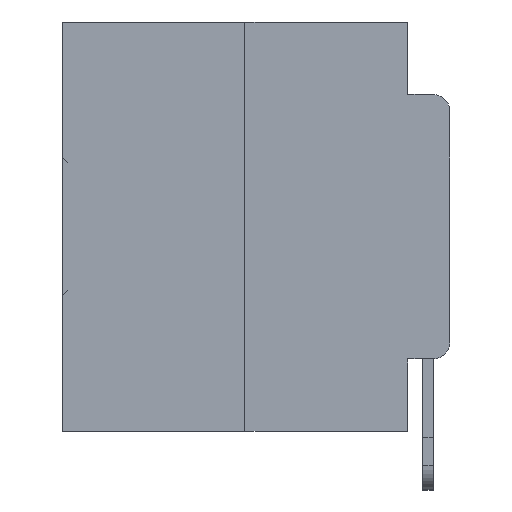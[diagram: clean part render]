
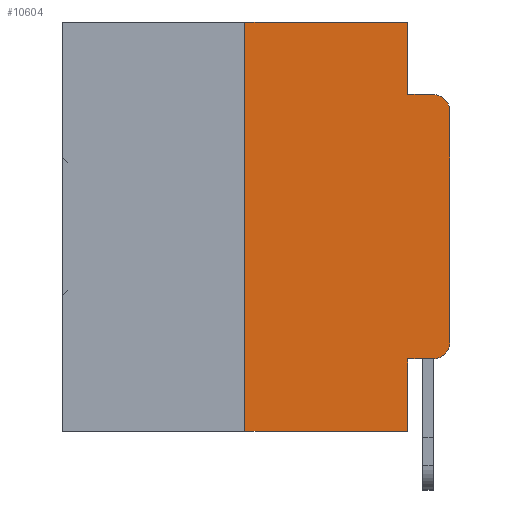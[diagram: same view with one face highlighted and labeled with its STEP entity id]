
A CAD part, left-side view. The second image highlights one B-rep face of the part: STEP entity #10604.
In plain terms, the highlighted planar face has unit normal (-1, 0, 0).
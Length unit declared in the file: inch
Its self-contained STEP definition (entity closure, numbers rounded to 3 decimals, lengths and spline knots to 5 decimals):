
#63 = LINE ( 'NONE', #8685, #33603 ) ;
#419 = DIRECTION ( 'NONE',  ( 0., -1., 0. ) ) ;
#886 = DIRECTION ( 'NONE',  ( 0., 0., -1. ) ) ;
#1869 = LINE ( 'NONE', #10910, #22253 ) ;
#2583 = ORIENTED_EDGE ( 'NONE', *, *, #24658, .F. ) ;
#2638 = VERTEX_POINT ( 'NONE', #23724 ) ;
#2683 = EDGE_CURVE ( 'NONE', #2638, #32949, #1869, .T. ) ;
#5233 = EDGE_CURVE ( 'NONE', #24261, #2638, #31438, .T. ) ;
#5281 = EDGE_CURVE ( 'NONE', #6270, #32305, #14330, .T. ) ;
#6270 = VERTEX_POINT ( 'NONE', #33329 ) ;
#7034 = EDGE_CURVE ( 'NONE', #11646, #24261, #29399, .T. ) ;
#7466 = ORIENTED_EDGE ( 'NONE', *, *, #28186, .F. ) ;
#7526 = AXIS2_PLACEMENT_3D ( 'NONE', #11898, #13704, #31930 ) ;
#8050 = VECTOR ( 'NONE', #419, 39.37008 ) ;
#8685 = CARTESIAN_POINT ( 'NONE',  ( 0., 0.25, 0. ) ) ;
#9119 = CARTESIAN_POINT ( 'NONE',  ( 0., 0.051, 0. ) ) ;
#9921 = ORIENTED_EDGE ( 'NONE', *, *, #7034, .T. ) ;
#10017 = CARTESIAN_POINT ( 'NONE',  ( 0., 0.051, -0.0885 ) ) ;
#10388 = CARTESIAN_POINT ( 'NONE',  ( 0., 0.25, -0.5 ) ) ;
#10493 = VECTOR ( 'NONE', #886, 39.37008 ) ;
#10604 = ADVANCED_FACE ( 'NONE', ( #17855 ), #31004, .F. ) ;
#10638 = DIRECTION ( 'NONE',  ( 0., -1., 0. ) ) ;
#10910 = CARTESIAN_POINT ( 'NONE',  ( 0., 0., 0. ) ) ;
#11521 = CARTESIAN_POINT ( 'NONE',  ( 0., 0.02, -0.1085 ) ) ;
#11646 = VERTEX_POINT ( 'NONE', #19890 ) ;
#11898 = CARTESIAN_POINT ( 'NONE',  ( 0., 0.02, -0.3915 ) ) ;
#12523 = DIRECTION ( 'NONE',  ( 0., 0., -1. ) ) ;
#12918 = LINE ( 'NONE', #21209, #24344 ) ;
#12978 = VERTEX_POINT ( 'NONE', #24254 ) ;
#13036 = ORIENTED_EDGE ( 'NONE', *, *, #5233, .T. ) ;
#13313 = DIRECTION ( 'NONE',  ( 0., 0., 1. ) ) ;
#13704 = DIRECTION ( 'NONE',  ( -1., 0., 0. ) ) ;
#14205 = DIRECTION ( 'NONE',  ( 0., 0., -1. ) ) ;
#14330 = LINE ( 'NONE', #16623, #8050 ) ;
#14402 = ORIENTED_EDGE ( 'NONE', *, *, #33355, .T. ) ;
#14422 = VECTOR ( 'NONE', #25820, 39.37008 ) ;
#14474 = CARTESIAN_POINT ( 'NONE',  ( 0., 0.051, -0.4115 ) ) ;
#15273 = VERTEX_POINT ( 'NONE', #19271 ) ;
#15423 = CARTESIAN_POINT ( 'NONE',  ( 0., 0.473, 0. ) ) ;
#15559 = VECTOR ( 'NONE', #30090, 39.37008 ) ;
#15974 = EDGE_CURVE ( 'NONE', #11646, #12978, #31324, .T. ) ;
#16623 = CARTESIAN_POINT ( 'NONE',  ( 0., 0.473, 0. ) ) ;
#16748 = DIRECTION ( 'NONE',  ( 0., 0., 1. ) ) ;
#17855 = FACE_OUTER_BOUND ( 'NONE', #27709, .T. ) ;
#17863 = CARTESIAN_POINT ( 'NONE',  ( 0., 0.051, 0. ) ) ;
#18067 = DIRECTION ( 'NONE',  ( 0., 0., -1. ) ) ;
#18108 = ORIENTED_EDGE ( 'NONE', *, *, #2683, .T. ) ;
#19271 = CARTESIAN_POINT ( 'NONE',  ( 0., 0.02, -0.0885 ) ) ;
#19890 = CARTESIAN_POINT ( 'NONE',  ( 0., 0.051, -0.4115 ) ) ;
#20770 = ORIENTED_EDGE ( 'NONE', *, *, #5281, .F. ) ;
#21209 = CARTESIAN_POINT ( 'NONE',  ( 0., 0.473, -0.5 ) ) ;
#21328 = CIRCLE ( 'NONE', #26271, 0.02 ) ;
#21358 = LINE ( 'NONE', #10017, #14422 ) ;
#21919 = CARTESIAN_POINT ( 'NONE',  ( 0., 0.051, -0.0885 ) ) ;
#22253 = VECTOR ( 'NONE', #13313, 39.37008 ) ;
#22598 = VECTOR ( 'NONE', #12523, 39.37008 ) ;
#22868 = AXIS2_PLACEMENT_3D ( 'NONE', #15423, #33546, #18067 ) ;
#22895 = CARTESIAN_POINT ( 'NONE',  ( 0., 0., -0.1085 ) ) ;
#23724 = CARTESIAN_POINT ( 'NONE',  ( 0., 0., -0.3915 ) ) ;
#23807 = EDGE_CURVE ( 'NONE', #29988, #12978, #12918, .T. ) ;
#24254 = CARTESIAN_POINT ( 'NONE',  ( 0., 0.051, -0.5 ) ) ;
#24261 = VERTEX_POINT ( 'NONE', #33408 ) ;
#24344 = VECTOR ( 'NONE', #10638, 39.37008 ) ;
#24658 = EDGE_CURVE ( 'NONE', #29988, #6270, #63, .T. ) ;
#24834 = ORIENTED_EDGE ( 'NONE', *, *, #26425, .F. ) ;
#25820 = DIRECTION ( 'NONE',  ( 0., -1., 0. ) ) ;
#26271 = AXIS2_PLACEMENT_3D ( 'NONE', #11521, #29829, #14205 ) ;
#26425 = EDGE_CURVE ( 'NONE', #32305, #28445, #30358, .T. ) ;
#27709 = EDGE_LOOP ( 'NONE', ( #18108, #14402, #7466, #24834, #20770, #2583, #32098, #29992, #9921, #13036 ) ) ;
#28186 = EDGE_CURVE ( 'NONE', #28445, #15273, #21358, .T. ) ;
#28445 = VERTEX_POINT ( 'NONE', #21919 ) ;
#29399 = LINE ( 'NONE', #14474, #15559 ) ;
#29829 = DIRECTION ( 'NONE',  ( -1., 0., 0. ) ) ;
#29988 = VERTEX_POINT ( 'NONE', #10388 ) ;
#29992 = ORIENTED_EDGE ( 'NONE', *, *, #15974, .F. ) ;
#30090 = DIRECTION ( 'NONE',  ( 0., -1., 0. ) ) ;
#30358 = LINE ( 'NONE', #17863, #22598 ) ;
#31004 = PLANE ( 'NONE',  #22868 ) ;
#31324 = LINE ( 'NONE', #9119, #10493 ) ;
#31438 = CIRCLE ( 'NONE', #7526, 0.02 ) ;
#31930 = DIRECTION ( 'NONE',  ( 0., 0., -1. ) ) ;
#32098 = ORIENTED_EDGE ( 'NONE', *, *, #23807, .T. ) ;
#32305 = VERTEX_POINT ( 'NONE', #32903 ) ;
#32903 = CARTESIAN_POINT ( 'NONE',  ( 0., 0.051, 0. ) ) ;
#32949 = VERTEX_POINT ( 'NONE', #22895 ) ;
#33329 = CARTESIAN_POINT ( 'NONE',  ( 0., 0.25, 0. ) ) ;
#33355 = EDGE_CURVE ( 'NONE', #32949, #15273, #21328, .T. ) ;
#33408 = CARTESIAN_POINT ( 'NONE',  ( 0., 0.02, -0.4115 ) ) ;
#33546 = DIRECTION ( 'NONE',  ( 1., 0., 0. ) ) ;
#33603 = VECTOR ( 'NONE', #16748, 39.37008 ) ;
